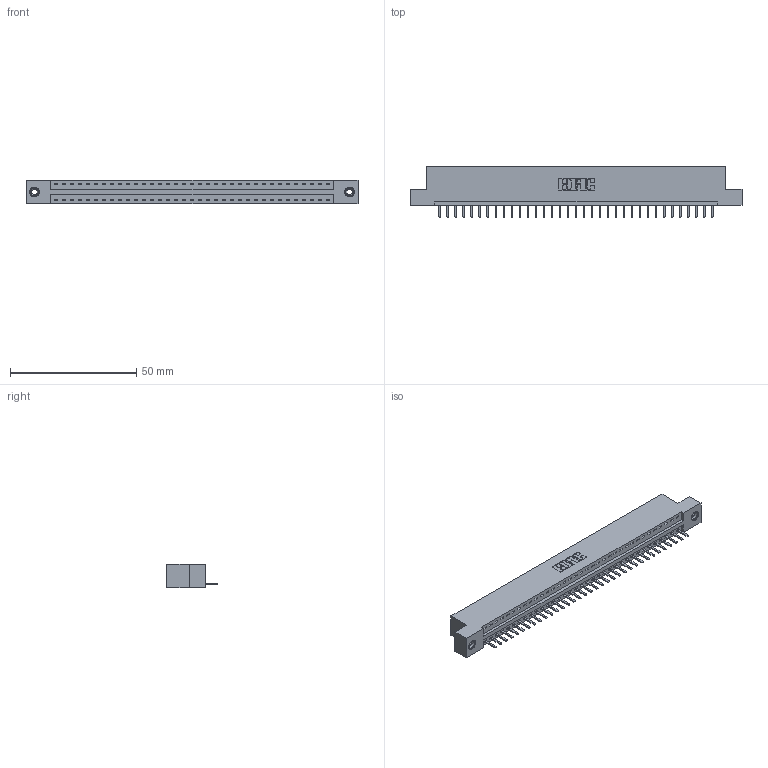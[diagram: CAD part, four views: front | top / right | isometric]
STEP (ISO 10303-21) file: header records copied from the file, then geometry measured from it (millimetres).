
FILE_DESCRIPTION (( 'STEP AP203' ), '1' );
FILE_NAME ('396-035-520-108.STEP', '2019-10-27T16:02:16', ( '' ), ( '' ), 'SwSTEP 2.0', 'SolidWorks 2016', '' );
FILE_SCHEMA (( 'CONFIG_CONTROL_DESIGN' ));
Length unit declared in the file: inch
Products named in the file (4): 345-250-001_345-250-003-102; 346 Part_Flush Mounting Lugs - 0.156 Dia-TI; 345-292-001_345-293-120; 396-035-520-108
Assembly tree (38 placements, depth 2):
  396-035-520-108
    346 Part_Flush Mounting Lugs - 0.156 Dia-TI
    345-292-001_345-293-120  x35
    345-250-001_345-250-003-102  x2
Bounding box: 131.7 x 20.02 x 9.4 mm (x, y, z)
Volume: 12451.1 mm3; surface area: 15172.4 mm2
Topology: 38 solids, 38 shells, 2352 faces, 6905 edges, 4502 vertices
Faces by surface type: plane 1578, cylinder 758, cone 12, torus 4
Entity records: 23964 total; most frequent: CARTESIAN_POINT 4104, ORIENTED_EDGE 4054, DIRECTION 3643, EDGE_CURVE 2027, LINE 1731, VECTOR 1731, VERTEX_POINT 1344, AXIS2_PLACEMENT_3D 956
